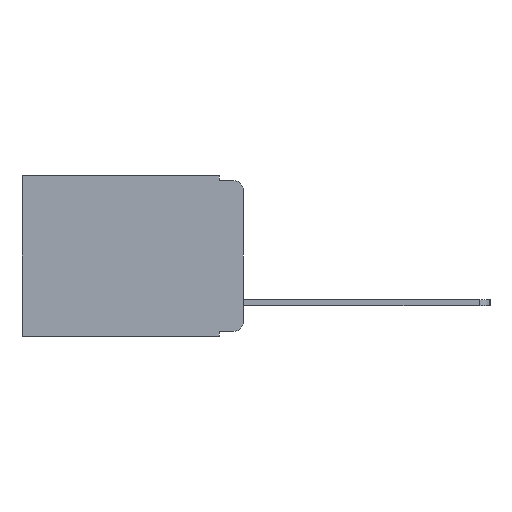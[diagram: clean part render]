
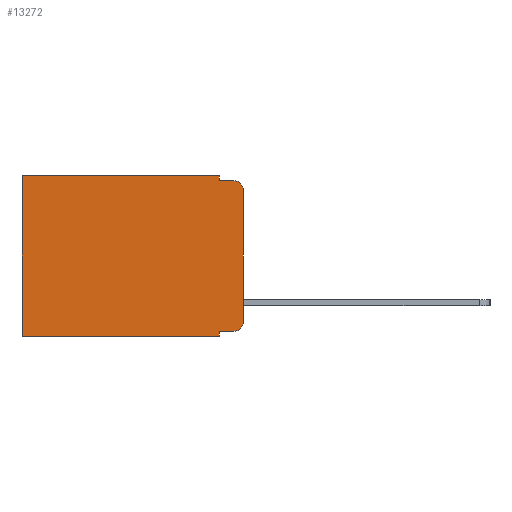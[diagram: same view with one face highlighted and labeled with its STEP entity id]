
A CAD part, left-side view. The second image highlights one B-rep face of the part: STEP entity #13272.
In plain terms, the highlighted planar face has unit normal (-1, 0, 0).
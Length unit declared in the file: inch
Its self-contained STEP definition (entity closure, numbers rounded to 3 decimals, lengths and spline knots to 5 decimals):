
#293 = DIRECTION ( 'NONE',  ( 1., 0., 0. ) ) ;
#336 = FACE_OUTER_BOUND ( 'NONE', #8427, .T. ) ;
#421 = EDGE_CURVE ( 'NONE', #21895, #13857, #3349, .T. ) ;
#449 = DIRECTION ( 'NONE',  ( 0., 1., 0. ) ) ;
#522 = DIRECTION ( 'NONE',  ( 0., -1., 0. ) ) ;
#824 = DIRECTION ( 'NONE',  ( -1., 0., 0. ) ) ;
#873 = VERTEX_POINT ( 'NONE', #20346 ) ;
#944 = CARTESIAN_POINT ( 'NONE',  ( 0.298, 0.051, -0.333 ) ) ;
#1505 = DIRECTION ( 'NONE',  ( 0., 0., -1. ) ) ;
#2792 = DIRECTION ( 'NONE',  ( -1., 0., 0. ) ) ;
#2804 = ORIENTED_EDGE ( 'NONE', *, *, #3281, .F. ) ;
#2968 = EDGE_CURVE ( 'NONE', #13857, #4110, #16763, .T. ) ;
#3281 = EDGE_CURVE ( 'NONE', #11844, #3813, #18288, .T. ) ;
#3349 = LINE ( 'NONE', #13517, #7091 ) ;
#3427 = CARTESIAN_POINT ( 'NONE',  ( 0.298, 0.051, -0.343 ) ) ;
#3760 = ORIENTED_EDGE ( 'NONE', *, *, #17836, .T. ) ;
#3813 = VERTEX_POINT ( 'NONE', #18874 ) ;
#4060 = ORIENTED_EDGE ( 'NONE', *, *, #421, .T. ) ;
#4098 = EDGE_CURVE ( 'NONE', #22141, #4433, #13402, .T. ) ;
#4110 = VERTEX_POINT ( 'NONE', #10242 ) ;
#4394 = AXIS2_PLACEMENT_3D ( 'NONE', #20947, #293, #12875 ) ;
#4433 = VERTEX_POINT ( 'NONE', #5946 ) ;
#4648 = DIRECTION ( 'NONE',  ( 0., -1., 0. ) ) ;
#4894 = DIRECTION ( 'NONE',  ( 0., 0., -1. ) ) ;
#5535 = CARTESIAN_POINT ( 'NONE',  ( 0.298, 0.02, -0.313 ) ) ;
#5646 = DIRECTION ( 'NONE',  ( 0., 1., 0. ) ) ;
#5812 = CARTESIAN_POINT ( 'NONE',  ( 0.298, 0.473, 0. ) ) ;
#5841 = CARTESIAN_POINT ( 'NONE',  ( 0.298, 0.051, 0. ) ) ;
#5946 = CARTESIAN_POINT ( 'NONE',  ( 0.298, 0.473, -0.343 ) ) ;
#7091 = VECTOR ( 'NONE', #4648, 39.37008 ) ;
#7438 = EDGE_CURVE ( 'NONE', #873, #4110, #15272, .T. ) ;
#7532 = VECTOR ( 'NONE', #9444, 39.37008 ) ;
#8236 = VERTEX_POINT ( 'NONE', #11289 ) ;
#8427 = EDGE_LOOP ( 'NONE', ( #10681, #21098, #16862, #2804, #19222, #3760, #15163, #19749, #4060, #18213 ) ) ;
#9444 = DIRECTION ( 'NONE',  ( 0., 0., -1. ) ) ;
#9477 = VECTOR ( 'NONE', #449, 39.37008 ) ;
#9509 = PLANE ( 'NONE',  #4394 ) ;
#10242 = CARTESIAN_POINT ( 'NONE',  ( 0.298, 0., -0.313 ) ) ;
#10681 = ORIENTED_EDGE ( 'NONE', *, *, #7438, .F. ) ;
#10889 = VECTOR ( 'NONE', #4894, 39.37008 ) ;
#11289 = CARTESIAN_POINT ( 'NONE',  ( 0.298, 0.02, -0.01 ) ) ;
#11414 = CARTESIAN_POINT ( 'NONE',  ( 0.298, 0.051, -0.01 ) ) ;
#11695 = VECTOR ( 'NONE', #5646, 39.37008 ) ;
#11765 = VECTOR ( 'NONE', #1505, 39.37008 ) ;
#11844 = VERTEX_POINT ( 'NONE', #5841 ) ;
#12141 = LINE ( 'NONE', #5812, #7532 ) ;
#12581 = CARTESIAN_POINT ( 'NONE',  ( 0.298, 0., 0. ) ) ;
#12875 = DIRECTION ( 'NONE',  ( 0., 0., -1. ) ) ;
#12987 = DIRECTION ( 'NONE',  ( 0., 0., -1. ) ) ;
#13029 = CARTESIAN_POINT ( 'NONE',  ( 0.298, 0.02, -0.333 ) ) ;
#13174 = EDGE_CURVE ( 'NONE', #11844, #17409, #16040, .T. ) ;
#13272 = ADVANCED_FACE ( 'NONE', ( #336 ), #9509, .F. ) ;
#13384 = CARTESIAN_POINT ( 'NONE',  ( 0.298, 0.02, -0.03 ) ) ;
#13402 = LINE ( 'NONE', #20943, #9477 ) ;
#13517 = CARTESIAN_POINT ( 'NONE',  ( 0.298, 0.051, -0.333 ) ) ;
#13857 = VERTEX_POINT ( 'NONE', #13029 ) ;
#15007 = DIRECTION ( 'NONE',  ( 0., 0., -1. ) ) ;
#15163 = ORIENTED_EDGE ( 'NONE', *, *, #4098, .F. ) ;
#15272 = LINE ( 'NONE', #18429, #10889 ) ;
#16040 = LINE ( 'NONE', #12581, #11695 ) ;
#16102 = LINE ( 'NONE', #21984, #11765 ) ;
#16258 = AXIS2_PLACEMENT_3D ( 'NONE', #13384, #2792, #15007 ) ;
#16753 = EDGE_CURVE ( 'NONE', #3813, #8236, #17033, .T. ) ;
#16763 = CIRCLE ( 'NONE', #19796, 0.02 ) ;
#16862 = ORIENTED_EDGE ( 'NONE', *, *, #16753, .F. ) ;
#17033 = LINE ( 'NONE', #11414, #21818 ) ;
#17409 = VERTEX_POINT ( 'NONE', #18171 ) ;
#17762 = VECTOR ( 'NONE', #21972, 39.37008 ) ;
#17836 = EDGE_CURVE ( 'NONE', #17409, #4433, #12141, .T. ) ;
#18171 = CARTESIAN_POINT ( 'NONE',  ( 0.298, 0.473, 0. ) ) ;
#18213 = ORIENTED_EDGE ( 'NONE', *, *, #2968, .T. ) ;
#18288 = LINE ( 'NONE', #22067, #17762 ) ;
#18429 = CARTESIAN_POINT ( 'NONE',  ( 0.298, 0., 0. ) ) ;
#18874 = CARTESIAN_POINT ( 'NONE',  ( 0.298, 0.051, -0.01 ) ) ;
#19222 = ORIENTED_EDGE ( 'NONE', *, *, #13174, .T. ) ;
#19749 = ORIENTED_EDGE ( 'NONE', *, *, #22129, .F. ) ;
#19796 = AXIS2_PLACEMENT_3D ( 'NONE', #5535, #824, #12987 ) ;
#20346 = CARTESIAN_POINT ( 'NONE',  ( 0.298, 0., -0.03 ) ) ;
#20676 = CIRCLE ( 'NONE', #16258, 0.02 ) ;
#20943 = CARTESIAN_POINT ( 'NONE',  ( 0.298, 0., -0.343 ) ) ;
#20947 = CARTESIAN_POINT ( 'NONE',  ( 0.298, 0., 0. ) ) ;
#21098 = ORIENTED_EDGE ( 'NONE', *, *, #21857, .T. ) ;
#21818 = VECTOR ( 'NONE', #522, 39.37008 ) ;
#21857 = EDGE_CURVE ( 'NONE', #873, #8236, #20676, .T. ) ;
#21895 = VERTEX_POINT ( 'NONE', #944 ) ;
#21972 = DIRECTION ( 'NONE',  ( 0., 0., -1. ) ) ;
#21984 = CARTESIAN_POINT ( 'NONE',  ( 0.298, 0.051, 0. ) ) ;
#22067 = CARTESIAN_POINT ( 'NONE',  ( 0.298, 0.051, 0. ) ) ;
#22129 = EDGE_CURVE ( 'NONE', #21895, #22141, #16102, .T. ) ;
#22141 = VERTEX_POINT ( 'NONE', #3427 ) ;
